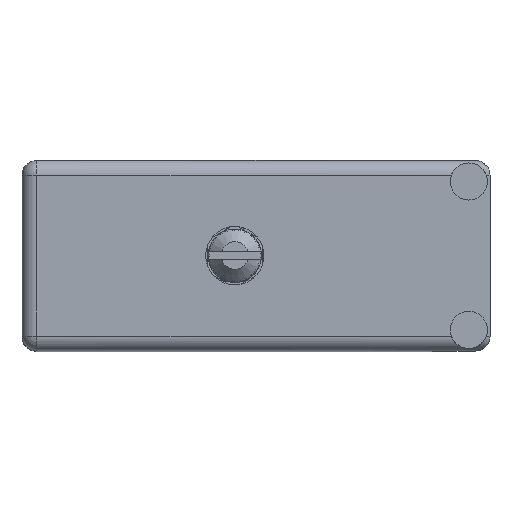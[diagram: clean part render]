
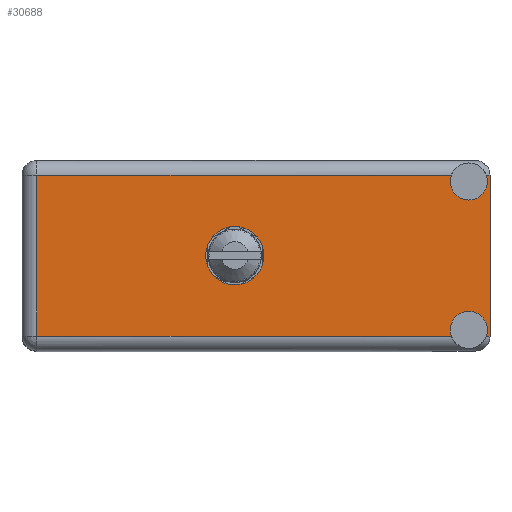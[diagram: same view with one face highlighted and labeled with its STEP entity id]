
A CAD part, top view. The second image highlights one B-rep face of the part: STEP entity #30688.
In plain terms, the highlighted face is planar.
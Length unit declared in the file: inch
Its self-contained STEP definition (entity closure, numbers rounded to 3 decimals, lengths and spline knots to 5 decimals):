
#629 = DIRECTION ( 'NONE',  ( 0., 1., 0. ) ) ;
#877 = CARTESIAN_POINT ( 'NONE',  ( 1.204, 1.466, 0.3795 ) ) ;
#1398 = EDGE_CURVE ( 'NONE', #95789, #90850, #16872, .T. ) ;
#3748 = CARTESIAN_POINT ( 'NONE',  ( 1.02162, 1.466, 0.3795 ) ) ;
#4750 = DIRECTION ( 'NONE',  ( 0., 0., 1. ) ) ;
#4950 = DIRECTION ( 'NONE',  ( 0., 0., 1. ) ) ;
#5144 = ORIENTED_EDGE ( 'NONE', *, *, #1398, .F. ) ;
#7337 = CARTESIAN_POINT ( 'NONE',  ( 0., 1.466, 0.1375 ) ) ;
#7395 = LINE ( 'NONE', #54437, #96722 ) ;
#11500 = ORIENTED_EDGE ( 'NONE', *, *, #71379, .F. ) ;
#11903 = DIRECTION ( 'NONE',  ( 0., 1., 0. ) ) ;
#14584 = EDGE_CURVE ( 'NONE', #55485, #42342, #34491, .T. ) ;
#14602 = DIRECTION ( 'NONE',  ( -1., 0., 0. ) ) ;
#14664 = DIRECTION ( 'NONE',  ( 0., 0., 1. ) ) ;
#14690 = DIRECTION ( 'NONE',  ( -1., 0., 0. ) ) ;
#15125 = LINE ( 'NONE', #64802, #80064 ) ;
#16378 = CARTESIAN_POINT ( 'NONE',  ( 0., 1.466, 0. ) ) ;
#16872 = CIRCLE ( 'NONE', #28841, 0.0875 ) ;
#17596 = EDGE_CURVE ( 'NONE', #88608, #74023, #15125, .T. ) ;
#17653 = EDGE_CURVE ( 'NONE', #81168, #74023, #42551, .T. ) ;
#18625 = CARTESIAN_POINT ( 'NONE',  ( 1.02162, 1.466, -0.3795 ) ) ;
#20085 = VECTOR ( 'NONE', #4750, 39.37008 ) ;
#20823 = AXIS2_PLACEMENT_3D ( 'NONE', #85179, #77694, #84661 ) ;
#21722 = VERTEX_POINT ( 'NONE', #88458 ) ;
#23912 = VECTOR ( 'NONE', #14690, 39.37008 ) ;
#24631 = ORIENTED_EDGE ( 'NONE', *, *, #14584, .F. ) ;
#24693 = DIRECTION ( 'NONE',  ( 0., 1., 0. ) ) ;
#27129 = CIRCLE ( 'NONE', #100448, 0.1375 ) ;
#27225 = CARTESIAN_POINT ( 'NONE',  ( -0.934, 1.466, -0.4495 ) ) ;
#28152 = VERTEX_POINT ( 'NONE', #18625 ) ;
#28405 = CARTESIAN_POINT ( 'NONE',  ( 1.204, 1.466, -0.3795 ) ) ;
#28841 = AXIS2_PLACEMENT_3D ( 'NONE', #65278, #24693, #43856 ) ;
#30688 = ADVANCED_FACE ( 'NONE', ( #48667, #104777 ), #80215, .T. ) ;
#31986 = ORIENTED_EDGE ( 'NONE', *, *, #17653, .F. ) ;
#34471 = DIRECTION ( 'NONE',  ( 0., 1., 0. ) ) ;
#34491 = CIRCLE ( 'NONE', #20823, 0.1375 ) ;
#35745 = AXIS2_PLACEMENT_3D ( 'NONE', #48232, #103287, #38626 ) ;
#38626 = DIRECTION ( 'NONE',  ( 0., 0., 1. ) ) ;
#38903 = DIRECTION ( 'NONE',  ( 1., 0., 0. ) ) ;
#40383 = EDGE_CURVE ( 'NONE', #90850, #84308, #60000, .T. ) ;
#40881 = DIRECTION ( 'NONE',  ( 0., 0., 1. ) ) ;
#42342 = VERTEX_POINT ( 'NONE', #105419 ) ;
#42551 = CIRCLE ( 'NONE', #35745, 0.0875 ) ;
#43679 = ORIENTED_EDGE ( 'NONE', *, *, #17596, .T. ) ;
#43856 = DIRECTION ( 'NONE',  ( 0., 0., 1. ) ) ;
#46739 = ORIENTED_EDGE ( 'NONE', *, *, #100024, .T. ) ;
#48232 = CARTESIAN_POINT ( 'NONE',  ( 1.104, 1.466, -0.35 ) ) ;
#48473 = ORIENTED_EDGE ( 'NONE', *, *, #59386, .T. ) ;
#48667 = FACE_BOUND ( 'NONE', #88739, .T. ) ;
#50249 = VERTEX_POINT ( 'NONE', #100608 ) ;
#54437 = CARTESIAN_POINT ( 'NONE',  ( 1.204, 1.466, 0.3795 ) ) ;
#54691 = VECTOR ( 'NONE', #14664, 39.37008 ) ;
#55485 = VERTEX_POINT ( 'NONE', #7337 ) ;
#55811 = LINE ( 'NONE', #103894, #23912 ) ;
#57996 = DIRECTION ( 'NONE',  ( 1., 0., 0. ) ) ;
#58964 = CARTESIAN_POINT ( 'NONE',  ( 1.104, 1.466, -0.2625 ) ) ;
#59386 = EDGE_CURVE ( 'NONE', #63702, #84308, #98583, .T. ) ;
#60000 = CIRCLE ( 'NONE', #75423, 0.0875 ) ;
#63702 = VERTEX_POINT ( 'NONE', #89464 ) ;
#64049 = CARTESIAN_POINT ( 'NONE',  ( 1.104, 1.466, 0.2625 ) ) ;
#64664 = AXIS2_PLACEMENT_3D ( 'NONE', #97813, #629, #80752 ) ;
#64802 = CARTESIAN_POINT ( 'NONE',  ( -1.004, 1.466, -0.3795 ) ) ;
#65194 = ORIENTED_EDGE ( 'NONE', *, *, #78880, .F. ) ;
#65278 = CARTESIAN_POINT ( 'NONE',  ( 1.104, 1.466, 0.35 ) ) ;
#65578 = ORIENTED_EDGE ( 'NONE', *, *, #40383, .F. ) ;
#66588 = ORIENTED_EDGE ( 'NONE', *, *, #74449, .T. ) ;
#68776 = EDGE_LOOP ( 'NONE', ( #48473, #65578, #5144, #46739, #65194, #43679, #31986, #84937, #66588, #72074 ) ) ;
#71379 = EDGE_CURVE ( 'NONE', #42342, #55485, #27129, .T. ) ;
#72074 = ORIENTED_EDGE ( 'NONE', *, *, #102522, .T. ) ;
#73088 = AXIS2_PLACEMENT_3D ( 'NONE', #91147, #34471, #40881 ) ;
#73550 = DIRECTION ( 'NONE',  ( 0., 0., 1. ) ) ;
#74023 = VERTEX_POINT ( 'NONE', #86569 ) ;
#74449 = EDGE_CURVE ( 'NONE', #28152, #50249, #55811, .T. ) ;
#74616 = DIRECTION ( 'NONE',  ( 0., 1., 0. ) ) ;
#75423 = AXIS2_PLACEMENT_3D ( 'NONE', #76046, #11903, #4950 ) ;
#76046 = CARTESIAN_POINT ( 'NONE',  ( 1.104, 1.466, 0.35 ) ) ;
#77694 = DIRECTION ( 'NONE',  ( 0., 1., 0. ) ) ;
#77953 = LINE ( 'NONE', #27225, #20085 ) ;
#78212 = CARTESIAN_POINT ( 'NONE',  ( 1.18638, 1.466, 0.3795 ) ) ;
#78880 = EDGE_CURVE ( 'NONE', #88608, #21722, #87887, .T. ) ;
#80064 = VECTOR ( 'NONE', #14602, 39.37008 ) ;
#80215 = PLANE ( 'NONE',  #64664 ) ;
#80370 = CARTESIAN_POINT ( 'NONE',  ( 1.204, 1.466, 0.4495 ) ) ;
#80752 = DIRECTION ( 'NONE',  ( -1., 0., 0. ) ) ;
#81168 = VERTEX_POINT ( 'NONE', #58964 ) ;
#84308 = VERTEX_POINT ( 'NONE', #3748 ) ;
#84661 = DIRECTION ( 'NONE',  ( 0., 0., 1. ) ) ;
#84937 = ORIENTED_EDGE ( 'NONE', *, *, #103919, .F. ) ;
#85179 = CARTESIAN_POINT ( 'NONE',  ( 0., 1.466, 0. ) ) ;
#86569 = CARTESIAN_POINT ( 'NONE',  ( 1.18638, 1.466, -0.3795 ) ) ;
#87887 = LINE ( 'NONE', #80370, #54691 ) ;
#88458 = CARTESIAN_POINT ( 'NONE',  ( 1.204, 1.466, 0.3795 ) ) ;
#88608 = VERTEX_POINT ( 'NONE', #28405 ) ;
#88739 = EDGE_LOOP ( 'NONE', ( #24631, #11500 ) ) ;
#89464 = CARTESIAN_POINT ( 'NONE',  ( -0.934, 1.466, 0.3795 ) ) ;
#90850 = VERTEX_POINT ( 'NONE', #64049 ) ;
#91147 = CARTESIAN_POINT ( 'NONE',  ( 1.104, 1.466, -0.35 ) ) ;
#95789 = VERTEX_POINT ( 'NONE', #78212 ) ;
#96722 = VECTOR ( 'NONE', #38903, 39.37008 ) ;
#97028 = CIRCLE ( 'NONE', #73088, 0.0875 ) ;
#97813 = CARTESIAN_POINT ( 'NONE',  ( -1.004, 1.466, -0.4495 ) ) ;
#98583 = LINE ( 'NONE', #877, #99940 ) ;
#99940 = VECTOR ( 'NONE', #57996, 39.37008 ) ;
#100024 = EDGE_CURVE ( 'NONE', #95789, #21722, #7395, .T. ) ;
#100448 = AXIS2_PLACEMENT_3D ( 'NONE', #16378, #74616, #73550 ) ;
#100608 = CARTESIAN_POINT ( 'NONE',  ( -0.934, 1.466, -0.3795 ) ) ;
#102522 = EDGE_CURVE ( 'NONE', #50249, #63702, #77953, .T. ) ;
#103287 = DIRECTION ( 'NONE',  ( 0., 1., 0. ) ) ;
#103894 = CARTESIAN_POINT ( 'NONE',  ( -1.004, 1.466, -0.3795 ) ) ;
#103919 = EDGE_CURVE ( 'NONE', #28152, #81168, #97028, .T. ) ;
#104777 = FACE_OUTER_BOUND ( 'NONE', #68776, .T. ) ;
#105419 = CARTESIAN_POINT ( 'NONE',  ( 0., 1.466, -0.1375 ) ) ;
